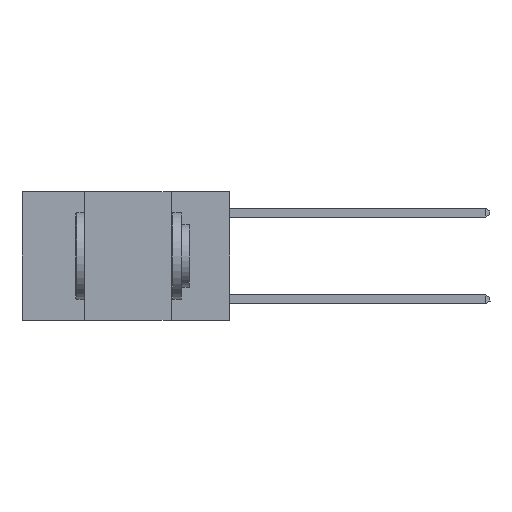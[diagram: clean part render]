
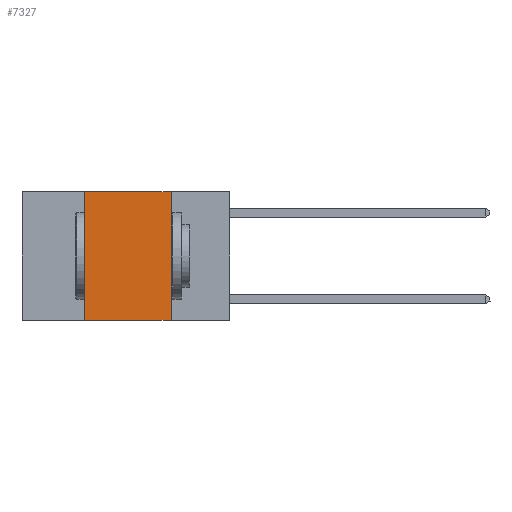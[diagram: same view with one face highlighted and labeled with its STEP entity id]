
A CAD part, left-side view. The second image highlights one B-rep face of the part: STEP entity #7327.
In plain terms, the highlighted planar face has unit normal (-1, 0, 0).
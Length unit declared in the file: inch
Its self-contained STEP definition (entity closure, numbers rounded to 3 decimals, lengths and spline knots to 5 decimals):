
#463 = CARTESIAN_POINT ( 'NONE',  ( 0., 0.17, 0. ) ) ;
#1257 = VERTEX_POINT ( 'NONE', #1356 ) ;
#1356 = CARTESIAN_POINT ( 'NONE',  ( 0., 0.17, -0.37 ) ) ;
#3284 = LINE ( 'NONE', #5531, #18251 ) ;
#3455 = LINE ( 'NONE', #14334, #17968 ) ;
#4473 = DIRECTION ( 'NONE',  ( 1., 0., 0. ) ) ;
#4517 = EDGE_CURVE ( 'NONE', #5964, #1257, #3455, .T. ) ;
#4730 = CARTESIAN_POINT ( 'NONE',  ( 0., 0.42, 0. ) ) ;
#4997 = LINE ( 'NONE', #4730, #12792 ) ;
#5294 = ORIENTED_EDGE ( 'NONE', *, *, #16981, .F. ) ;
#5531 = CARTESIAN_POINT ( 'NONE',  ( 0., 0.17, 0. ) ) ;
#5917 = DIRECTION ( 'NONE',  ( 0., -1., 0. ) ) ;
#5964 = VERTEX_POINT ( 'NONE', #17308 ) ;
#7327 = ADVANCED_FACE ( 'NONE', ( #14566 ), #10330, .F. ) ;
#7437 = EDGE_CURVE ( 'NONE', #5964, #13822, #4997, .T. ) ;
#8208 = LINE ( 'NONE', #17453, #15428 ) ;
#9276 = EDGE_CURVE ( 'NONE', #10359, #1257, #3284, .T. ) ;
#9522 = EDGE_LOOP ( 'NONE', ( #12191, #5294, #18202, #11365 ) ) ;
#10330 = PLANE ( 'NONE',  #12472 ) ;
#10359 = VERTEX_POINT ( 'NONE', #463 ) ;
#11365 = ORIENTED_EDGE ( 'NONE', *, *, #4517, .T. ) ;
#11793 = CARTESIAN_POINT ( 'NONE',  ( 0., 0.6, 0. ) ) ;
#12191 = ORIENTED_EDGE ( 'NONE', *, *, #9276, .F. ) ;
#12472 = AXIS2_PLACEMENT_3D ( 'NONE', #11793, #4473, #14662 ) ;
#12792 = VECTOR ( 'NONE', #17679, 39.37008 ) ;
#13822 = VERTEX_POINT ( 'NONE', #15558 ) ;
#14334 = CARTESIAN_POINT ( 'NONE',  ( 0., 0.6, -0.37 ) ) ;
#14566 = FACE_OUTER_BOUND ( 'NONE', #9522, .T. ) ;
#14662 = DIRECTION ( 'NONE',  ( 0., 0., -1. ) ) ;
#15428 = VECTOR ( 'NONE', #5917, 39.37008 ) ;
#15558 = CARTESIAN_POINT ( 'NONE',  ( 0., 0.42, 0. ) ) ;
#15765 = DIRECTION ( 'NONE',  ( 0., -1., 0. ) ) ;
#16981 = EDGE_CURVE ( 'NONE', #13822, #10359, #8208, .T. ) ;
#17308 = CARTESIAN_POINT ( 'NONE',  ( 0., 0.42, -0.37 ) ) ;
#17453 = CARTESIAN_POINT ( 'NONE',  ( 0., 0.6, 0. ) ) ;
#17679 = DIRECTION ( 'NONE',  ( 0., 0., 1. ) ) ;
#17968 = VECTOR ( 'NONE', #15765, 39.37008 ) ;
#18202 = ORIENTED_EDGE ( 'NONE', *, *, #7437, .F. ) ;
#18251 = VECTOR ( 'NONE', #18482, 39.37008 ) ;
#18482 = DIRECTION ( 'NONE',  ( 0., 0., -1. ) ) ;
